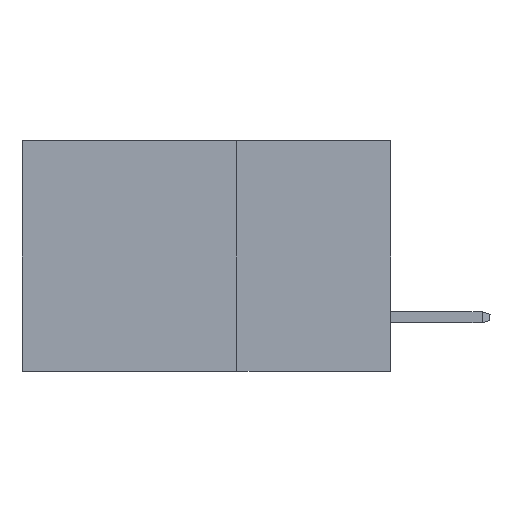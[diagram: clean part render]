
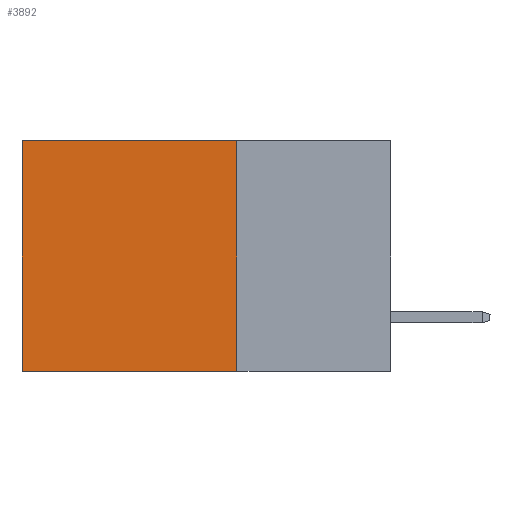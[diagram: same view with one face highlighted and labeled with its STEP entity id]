
A CAD part, left-side view. The second image highlights one B-rep face of the part: STEP entity #3892.
In plain terms, the highlighted planar face has unit normal (-1, 0, 0).
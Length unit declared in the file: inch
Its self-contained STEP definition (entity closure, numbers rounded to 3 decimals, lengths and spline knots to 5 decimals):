
#156 = LINE ( 'NONE', #2221, #7828 ) ;
#701 = VECTOR ( 'NONE', #12754, 39.37008 ) ;
#1103 = EDGE_CURVE ( 'NONE', #3868, #10341, #9398, .T. ) ;
#1626 = ORIENTED_EDGE ( 'NONE', *, *, #7151, .T. ) ;
#2221 = CARTESIAN_POINT ( 'NONE',  ( 0.2875, 0.6, -0.375 ) ) ;
#2317 = VECTOR ( 'NONE', #7210, 39.37008 ) ;
#2426 = ORIENTED_EDGE ( 'NONE', *, *, #4048, .F. ) ;
#2599 = ORIENTED_EDGE ( 'NONE', *, *, #9436, .T. ) ;
#2659 = PLANE ( 'NONE',  #10649 ) ;
#2869 = CARTESIAN_POINT ( 'NONE',  ( 0.2875, 0.25, -0.375 ) ) ;
#3579 = EDGE_LOOP ( 'NONE', ( #2599, #11321, #2426, #1626 ) ) ;
#3868 = VERTEX_POINT ( 'NONE', #2869 ) ;
#3892 = ADVANCED_FACE ( 'NONE', ( #7821 ), #2659, .F. ) ;
#4048 = EDGE_CURVE ( 'NONE', #12599, #3868, #9148, .T. ) ;
#4253 = DIRECTION ( 'NONE',  ( 0., 1., 0. ) ) ;
#4812 = DIRECTION ( 'NONE',  ( 1., 0., 0. ) ) ;
#5180 = DIRECTION ( 'NONE',  ( 0., 0., -1. ) ) ;
#5761 = CARTESIAN_POINT ( 'NONE',  ( 0.2875, 0.6, 0. ) ) ;
#6598 = LINE ( 'NONE', #12554, #701 ) ;
#6755 = DIRECTION ( 'NONE',  ( 0., 0., -1. ) ) ;
#7020 = CARTESIAN_POINT ( 'NONE',  ( 0.2875, 0.25, -0.375 ) ) ;
#7151 = EDGE_CURVE ( 'NONE', #12599, #12065, #6598, .T. ) ;
#7210 = DIRECTION ( 'NONE',  ( 0., 0., -1. ) ) ;
#7263 = CARTESIAN_POINT ( 'NONE',  ( 0.2875, 0.25, -0.375 ) ) ;
#7821 = FACE_OUTER_BOUND ( 'NONE', #3579, .T. ) ;
#7828 = VECTOR ( 'NONE', #5180, 39.37008 ) ;
#8753 = CARTESIAN_POINT ( 'NONE',  ( 0.2875, 0.25, -0.375 ) ) ;
#9148 = LINE ( 'NONE', #7020, #2317 ) ;
#9398 = LINE ( 'NONE', #7263, #9569 ) ;
#9436 = EDGE_CURVE ( 'NONE', #12065, #10341, #156, .T. ) ;
#9569 = VECTOR ( 'NONE', #4253, 39.37008 ) ;
#10341 = VERTEX_POINT ( 'NONE', #13190 ) ;
#10649 = AXIS2_PLACEMENT_3D ( 'NONE', #8753, #4812, #6755 ) ;
#10832 = CARTESIAN_POINT ( 'NONE',  ( 0.2875, 0.25, 0. ) ) ;
#11321 = ORIENTED_EDGE ( 'NONE', *, *, #1103, .F. ) ;
#12065 = VERTEX_POINT ( 'NONE', #5761 ) ;
#12554 = CARTESIAN_POINT ( 'NONE',  ( 0.2875, 0.25, 0. ) ) ;
#12599 = VERTEX_POINT ( 'NONE', #10832 ) ;
#12754 = DIRECTION ( 'NONE',  ( 0., 1., 0. ) ) ;
#13190 = CARTESIAN_POINT ( 'NONE',  ( 0.2875, 0.6, -0.375 ) ) ;
